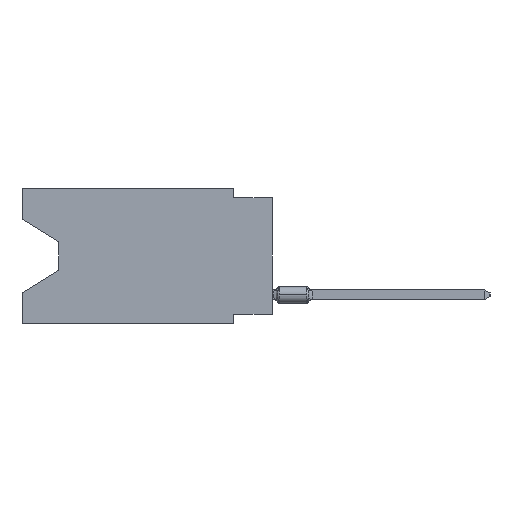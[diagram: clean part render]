
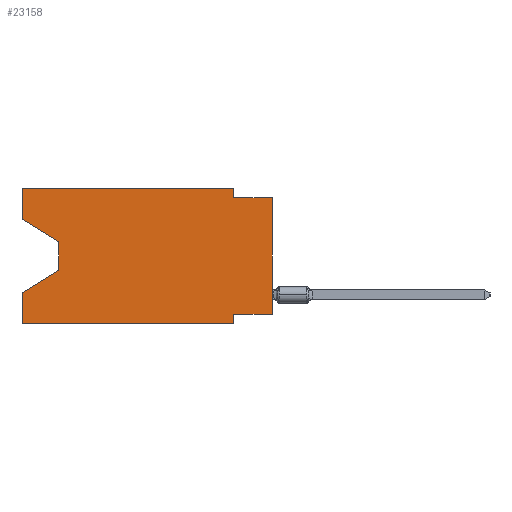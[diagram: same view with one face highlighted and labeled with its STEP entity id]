
A CAD part, left-side view. The second image highlights one B-rep face of the part: STEP entity #23158.
In plain terms, the highlighted planar face has unit normal (-1, 0, 0).
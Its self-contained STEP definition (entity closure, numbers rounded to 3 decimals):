
#326 = VECTOR ( 'NONE', #16856, 1000. ) ;
#1487 = ORIENTED_EDGE ( 'NONE', *, *, #5900, .F. ) ;
#1539 = ORIENTED_EDGE ( 'NONE', *, *, #22683, .T. ) ;
#1742 = DIRECTION ( 'NONE',  ( 0., -1., 0. ) ) ;
#3206 = VERTEX_POINT ( 'NONE', #37842 ) ;
#3574 = CARTESIAN_POINT ( 'NONE',  ( 0., 16.383, -6.852 ) ) ;
#3702 = LINE ( 'NONE', #15867, #7185 ) ;
#3841 = ORIENTED_EDGE ( 'NONE', *, *, #11183, .T. ) ;
#4125 = CARTESIAN_POINT ( 'NONE',  ( 0., 2.54, -0.635 ) ) ;
#4526 = VECTOR ( 'NONE', #17315, 1000. ) ;
#4803 = EDGE_CURVE ( 'NONE', #28669, #19326, #37883, .T. ) ;
#5355 = CARTESIAN_POINT ( 'NONE',  ( 0., 16.383, -2.038 ) ) ;
#5900 = EDGE_CURVE ( 'NONE', #24284, #30825, #21327, .T. ) ;
#5910 = VERTEX_POINT ( 'NONE', #13180 ) ;
#6407 = PLANE ( 'NONE',  #32514 ) ;
#6501 = ORIENTED_EDGE ( 'NONE', *, *, #29963, .F. ) ;
#6510 = ORIENTED_EDGE ( 'NONE', *, *, #15336, .F. ) ;
#6994 = VECTOR ( 'NONE', #34925, 1000. ) ;
#7011 = DIRECTION ( 'NONE',  ( 0., 0.855, -0.519 ) ) ;
#7068 = CARTESIAN_POINT ( 'NONE',  ( 0., 0., 0. ) ) ;
#7162 = VERTEX_POINT ( 'NONE', #7918 ) ;
#7185 = VECTOR ( 'NONE', #16060, 1000. ) ;
#7585 = LINE ( 'NONE', #32262, #326 ) ;
#7652 = EDGE_CURVE ( 'NONE', #3206, #11614, #11308, .T. ) ;
#7918 = CARTESIAN_POINT ( 'NONE',  ( 0., 13.97, -3.505 ) ) ;
#7948 = VECTOR ( 'NONE', #20195, 1000. ) ;
#8185 = LINE ( 'NONE', #19986, #27830 ) ;
#8841 = VECTOR ( 'NONE', #12432, 1000. ) ;
#9453 = ORIENTED_EDGE ( 'NONE', *, *, #4803, .T. ) ;
#9838 = VERTEX_POINT ( 'NONE', #5355 ) ;
#10130 = CARTESIAN_POINT ( 'NONE',  ( 0., 0., -0.635 ) ) ;
#10504 = VERTEX_POINT ( 'NONE', #3574 ) ;
#10541 = LINE ( 'NONE', #7068, #32775 ) ;
#11123 = CARTESIAN_POINT ( 'NONE',  ( 0., 2.54, 0. ) ) ;
#11183 = EDGE_CURVE ( 'NONE', #7162, #20456, #23344, .T. ) ;
#11308 = LINE ( 'NONE', #23104, #7948 ) ;
#11600 = EDGE_CURVE ( 'NONE', #11614, #27980, #31611, .T. ) ;
#11614 = VERTEX_POINT ( 'NONE', #28526 ) ;
#12270 = ORIENTED_EDGE ( 'NONE', *, *, #17952, .F. ) ;
#12432 = DIRECTION ( 'NONE',  ( 0., 1., 0. ) ) ;
#13180 = CARTESIAN_POINT ( 'NONE',  ( 0., 0., -0.635 ) ) ;
#15108 = CARTESIAN_POINT ( 'NONE',  ( 0., 16.383, 0. ) ) ;
#15298 = FACE_OUTER_BOUND ( 'NONE', #18956, .T. ) ;
#15336 = EDGE_CURVE ( 'NONE', #28669, #10504, #7585, .T. ) ;
#15772 = CARTESIAN_POINT ( 'NONE',  ( 0., 0., -8.255 ) ) ;
#15867 = CARTESIAN_POINT ( 'NONE',  ( 0., 2.54, -8.89 ) ) ;
#16060 = DIRECTION ( 'NONE',  ( 0., 0., -1. ) ) ;
#16856 = DIRECTION ( 'NONE',  ( 0., 0., 1. ) ) ;
#17315 = DIRECTION ( 'NONE',  ( 0., 0., -1. ) ) ;
#17952 = EDGE_CURVE ( 'NONE', #9838, #3206, #18465, .T. ) ;
#18465 = LINE ( 'NONE', #21936, #28469 ) ;
#18869 = CARTESIAN_POINT ( 'NONE',  ( 0., 13.97, -5.385 ) ) ;
#18956 = EDGE_LOOP ( 'NONE', ( #1539, #3841, #34414, #6510, #9453, #33586, #1487, #25011, #6501, #29807, #20411, #12270 ) ) ;
#18977 = CARTESIAN_POINT ( 'NONE',  ( 0., 0., -8.255 ) ) ;
#19326 = VERTEX_POINT ( 'NONE', #32399 ) ;
#19424 = EDGE_CURVE ( 'NONE', #24284, #5910, #10541, .T. ) ;
#19986 = CARTESIAN_POINT ( 'NONE',  ( 0., 16.383, -2.038 ) ) ;
#20195 = DIRECTION ( 'NONE',  ( 0., -1., 0. ) ) ;
#20411 = ORIENTED_EDGE ( 'NONE', *, *, #7652, .F. ) ;
#20456 = VERTEX_POINT ( 'NONE', #18869 ) ;
#21327 = LINE ( 'NONE', #18977, #8841 ) ;
#21334 = LINE ( 'NONE', #33672, #26918 ) ;
#21936 = CARTESIAN_POINT ( 'NONE',  ( 0., 16.383, 0. ) ) ;
#22106 = VECTOR ( 'NONE', #27728, 1000. ) ;
#22122 = DIRECTION ( 'NONE',  ( 0., 0., 1. ) ) ;
#22683 = EDGE_CURVE ( 'NONE', #9838, #7162, #8185, .T. ) ;
#23104 = CARTESIAN_POINT ( 'NONE',  ( 0., 16.383, 0. ) ) ;
#23158 = ADVANCED_FACE ( 'NONE', ( #15298 ), #6407, .F. ) ;
#23344 = LINE ( 'NONE', #31454, #6994 ) ;
#24284 = VERTEX_POINT ( 'NONE', #15772 ) ;
#24494 = DIRECTION ( 'NONE',  ( 0., 0., 1. ) ) ;
#25011 = ORIENTED_EDGE ( 'NONE', *, *, #19424, .T. ) ;
#26709 = VECTOR ( 'NONE', #1742, 1000. ) ;
#26918 = VECTOR ( 'NONE', #7011, 1000. ) ;
#27728 = DIRECTION ( 'NONE',  ( 0., -1., 0. ) ) ;
#27830 = VECTOR ( 'NONE', #31768, 1000. ) ;
#27980 = VERTEX_POINT ( 'NONE', #4125 ) ;
#28239 = CARTESIAN_POINT ( 'NONE',  ( 0., 16.383, -8.89 ) ) ;
#28469 = VECTOR ( 'NONE', #22122, 1000. ) ;
#28526 = CARTESIAN_POINT ( 'NONE',  ( 0., 2.54, 0. ) ) ;
#28669 = VERTEX_POINT ( 'NONE', #34951 ) ;
#29799 = DIRECTION ( 'NONE',  ( 1., 0., 0. ) ) ;
#29807 = ORIENTED_EDGE ( 'NONE', *, *, #11600, .F. ) ;
#29963 = EDGE_CURVE ( 'NONE', #27980, #5910, #34074, .T. ) ;
#30825 = VERTEX_POINT ( 'NONE', #38170 ) ;
#31454 = CARTESIAN_POINT ( 'NONE',  ( 0., 13.97, -3.505 ) ) ;
#31611 = LINE ( 'NONE', #11123, #4526 ) ;
#31768 = DIRECTION ( 'NONE',  ( 0., -0.855, -0.519 ) ) ;
#31991 = EDGE_CURVE ( 'NONE', #20456, #10504, #21334, .T. ) ;
#32262 = CARTESIAN_POINT ( 'NONE',  ( 0., 16.383, 0. ) ) ;
#32399 = CARTESIAN_POINT ( 'NONE',  ( 0., 2.54, -8.89 ) ) ;
#32493 = DIRECTION ( 'NONE',  ( 0., 0., -1. ) ) ;
#32514 = AXIS2_PLACEMENT_3D ( 'NONE', #15108, #29799, #32493 ) ;
#32775 = VECTOR ( 'NONE', #24494, 1000. ) ;
#33586 = ORIENTED_EDGE ( 'NONE', *, *, #34703, .F. ) ;
#33672 = CARTESIAN_POINT ( 'NONE',  ( 0., 13.97, -5.385 ) ) ;
#34074 = LINE ( 'NONE', #10130, #22106 ) ;
#34414 = ORIENTED_EDGE ( 'NONE', *, *, #31991, .T. ) ;
#34703 = EDGE_CURVE ( 'NONE', #30825, #19326, #3702, .T. ) ;
#34925 = DIRECTION ( 'NONE',  ( 0., 0., -1. ) ) ;
#34951 = CARTESIAN_POINT ( 'NONE',  ( 0., 16.383, -8.89 ) ) ;
#37842 = CARTESIAN_POINT ( 'NONE',  ( 0., 16.383, 0. ) ) ;
#37883 = LINE ( 'NONE', #28239, #26709 ) ;
#38170 = CARTESIAN_POINT ( 'NONE',  ( 0., 2.54, -8.255 ) ) ;
